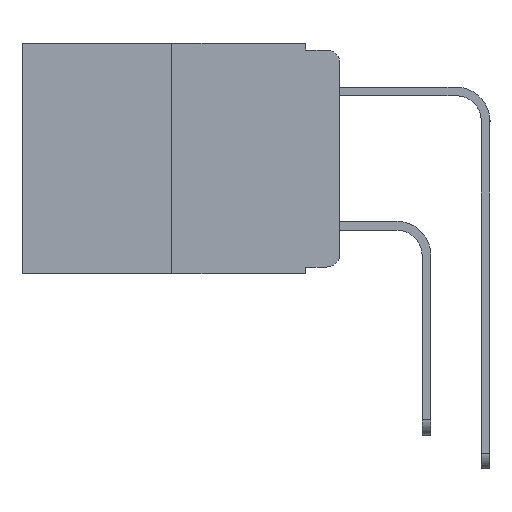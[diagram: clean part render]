
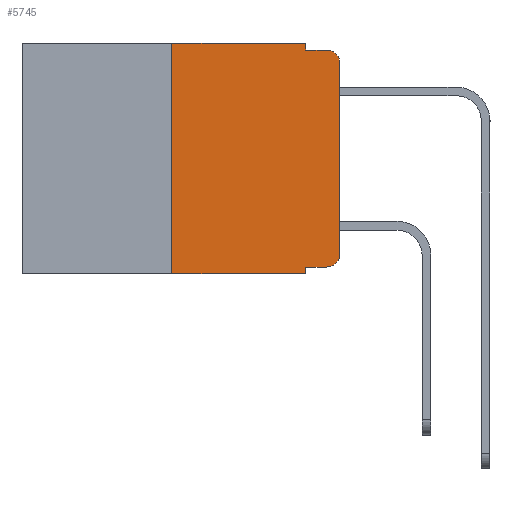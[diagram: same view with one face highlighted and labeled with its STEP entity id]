
A CAD part, left-side view. The second image highlights one B-rep face of the part: STEP entity #5745.
In plain terms, the highlighted planar face has unit normal (-1, 0, 0).
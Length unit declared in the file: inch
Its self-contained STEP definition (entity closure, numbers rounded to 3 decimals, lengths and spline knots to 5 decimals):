
#398 = PLANE ( 'NONE',  #7154 ) ;
#621 = EDGE_CURVE ( 'NONE', #5343, #4129, #8855, .T. ) ;
#921 = FACE_OUTER_BOUND ( 'NONE', #2505, .T. ) ;
#965 = EDGE_CURVE ( 'NONE', #5343, #5783, #12676, .T. ) ;
#1236 = CARTESIAN_POINT ( 'NONE',  ( 0., 0., 0. ) ) ;
#1348 = CARTESIAN_POINT ( 'NONE',  ( 0., 0.051, 0. ) ) ;
#1550 = ORIENTED_EDGE ( 'NONE', *, *, #5562, .T. ) ;
#1567 = CARTESIAN_POINT ( 'NONE',  ( 0., 0.02, -0.03 ) ) ;
#1659 = DIRECTION ( 'NONE',  ( 0., 0., -1. ) ) ;
#1969 = ORIENTED_EDGE ( 'NONE', *, *, #5755, .T. ) ;
#2050 = ORIENTED_EDGE ( 'NONE', *, *, #6531, .F. ) ;
#2222 = ORIENTED_EDGE ( 'NONE', *, *, #3668, .F. ) ;
#2332 = ORIENTED_EDGE ( 'NONE', *, *, #12417, .F. ) ;
#2345 = ORIENTED_EDGE ( 'NONE', *, *, #621, .F. ) ;
#2492 = VERTEX_POINT ( 'NONE', #4375 ) ;
#2505 = EDGE_LOOP ( 'NONE', ( #1550, #1969, #2050, #2222, #2332, #2345, #2548, #2561, #3555, #4315 ) ) ;
#2548 = ORIENTED_EDGE ( 'NONE', *, *, #965, .T. ) ;
#2561 = ORIENTED_EDGE ( 'NONE', *, *, #13396, .F. ) ;
#2664 = DIRECTION ( 'NONE',  ( 0., 0., -1. ) ) ;
#2717 = DIRECTION ( 'NONE',  ( 0., 0., -1. ) ) ;
#3131 = CARTESIAN_POINT ( 'NONE',  ( 0., 0.25, -0.343 ) ) ;
#3384 = LINE ( 'NONE', #10228, #6253 ) ;
#3555 = ORIENTED_EDGE ( 'NONE', *, *, #12103, .T. ) ;
#3668 = EDGE_CURVE ( 'NONE', #4935, #10094, #12085, .T. ) ;
#3750 = VECTOR ( 'NONE', #13242, 39.37008 ) ;
#3945 = CARTESIAN_POINT ( 'NONE',  ( 0., 0.25, 0. ) ) ;
#4071 = DIRECTION ( 'NONE',  ( 0., -1., 0. ) ) ;
#4129 = VERTEX_POINT ( 'NONE', #5548 ) ;
#4315 = ORIENTED_EDGE ( 'NONE', *, *, #8825, .T. ) ;
#4375 = CARTESIAN_POINT ( 'NONE',  ( 0., 0., -0.313 ) ) ;
#4385 = VERTEX_POINT ( 'NONE', #12910 ) ;
#4935 = VERTEX_POINT ( 'NONE', #1348 ) ;
#5325 = DIRECTION ( 'NONE',  ( 0., 0., -1. ) ) ;
#5343 = VERTEX_POINT ( 'NONE', #3131 ) ;
#5548 = CARTESIAN_POINT ( 'NONE',  ( 0., 0.25, 0. ) ) ;
#5562 = EDGE_CURVE ( 'NONE', #2492, #11423, #5974, .T. ) ;
#5582 = DIRECTION ( 'NONE',  ( 0., 0., 1. ) ) ;
#5693 = CARTESIAN_POINT ( 'NONE',  ( 0., 0.473, 0. ) ) ;
#5741 = CARTESIAN_POINT ( 'NONE',  ( 0., 0.051, -0.333 ) ) ;
#5745 = ADVANCED_FACE ( 'NONE', ( #921 ), #398, .F. ) ;
#5755 = EDGE_CURVE ( 'NONE', #11423, #4385, #6756, .T. ) ;
#5783 = VERTEX_POINT ( 'NONE', #10031 ) ;
#5974 = LINE ( 'NONE', #1236, #10977 ) ;
#6021 = DIRECTION ( 'NONE',  ( -1., 0., 0. ) ) ;
#6111 = CARTESIAN_POINT ( 'NONE',  ( 0., 0., -0.03 ) ) ;
#6253 = VECTOR ( 'NONE', #4071, 39.37008 ) ;
#6326 = CARTESIAN_POINT ( 'NONE',  ( 0., 0.051, -0.01 ) ) ;
#6470 = AXIS2_PLACEMENT_3D ( 'NONE', #1567, #9040, #2717 ) ;
#6497 = CIRCLE ( 'NONE', #12001, 0.02 ) ;
#6531 = EDGE_CURVE ( 'NONE', #10094, #4385, #12922, .T. ) ;
#6756 = CIRCLE ( 'NONE', #6470, 0.02 ) ;
#6832 = DIRECTION ( 'NONE',  ( 0., -1., 0. ) ) ;
#7154 = AXIS2_PLACEMENT_3D ( 'NONE', #7975, #8984, #2664 ) ;
#7765 = CARTESIAN_POINT ( 'NONE',  ( 0., 0.02, -0.333 ) ) ;
#7975 = CARTESIAN_POINT ( 'NONE',  ( 0., 0.473, 0. ) ) ;
#7998 = VERTEX_POINT ( 'NONE', #7765 ) ;
#8587 = VECTOR ( 'NONE', #5325, 39.37008 ) ;
#8655 = CARTESIAN_POINT ( 'NONE',  ( 0., 0.051, 0. ) ) ;
#8743 = DIRECTION ( 'NONE',  ( 0., 0., 1. ) ) ;
#8825 = EDGE_CURVE ( 'NONE', #7998, #2492, #6497, .T. ) ;
#8855 = LINE ( 'NONE', #3945, #10863 ) ;
#8984 = DIRECTION ( 'NONE',  ( 1., 0., 0. ) ) ;
#9040 = DIRECTION ( 'NONE',  ( -1., 0., 0. ) ) ;
#9771 = VECTOR ( 'NONE', #6832, 39.37008 ) ;
#9942 = CARTESIAN_POINT ( 'NONE',  ( 0., 0.051, -0.01 ) ) ;
#10031 = CARTESIAN_POINT ( 'NONE',  ( 0., 0.051, -0.343 ) ) ;
#10094 = VERTEX_POINT ( 'NONE', #9942 ) ;
#10175 = LINE ( 'NONE', #5693, #10789 ) ;
#10228 = CARTESIAN_POINT ( 'NONE',  ( 0., 0.051, -0.333 ) ) ;
#10789 = VECTOR ( 'NONE', #11662, 39.37008 ) ;
#10863 = VECTOR ( 'NONE', #5582, 39.37008 ) ;
#10977 = VECTOR ( 'NONE', #8743, 39.37008 ) ;
#11201 = LINE ( 'NONE', #11338, #8587 ) ;
#11338 = CARTESIAN_POINT ( 'NONE',  ( 0., 0.051, 0. ) ) ;
#11423 = VERTEX_POINT ( 'NONE', #6111 ) ;
#11662 = DIRECTION ( 'NONE',  ( 0., -1., 0. ) ) ;
#11775 = VECTOR ( 'NONE', #1659, 39.37008 ) ;
#11970 = CARTESIAN_POINT ( 'NONE',  ( 0., 0.02, -0.313 ) ) ;
#12001 = AXIS2_PLACEMENT_3D ( 'NONE', #11970, #6021, #12946 ) ;
#12085 = LINE ( 'NONE', #8655, #11775 ) ;
#12103 = EDGE_CURVE ( 'NONE', #12454, #7998, #3384, .T. ) ;
#12417 = EDGE_CURVE ( 'NONE', #4129, #4935, #10175, .T. ) ;
#12454 = VERTEX_POINT ( 'NONE', #5741 ) ;
#12676 = LINE ( 'NONE', #12868, #9771 ) ;
#12868 = CARTESIAN_POINT ( 'NONE',  ( 0., 0.473, -0.343 ) ) ;
#12910 = CARTESIAN_POINT ( 'NONE',  ( 0., 0.02, -0.01 ) ) ;
#12922 = LINE ( 'NONE', #6326, #3750 ) ;
#12946 = DIRECTION ( 'NONE',  ( 0., 0., -1. ) ) ;
#13242 = DIRECTION ( 'NONE',  ( 0., -1., 0. ) ) ;
#13396 = EDGE_CURVE ( 'NONE', #12454, #5783, #11201, .T. ) ;
